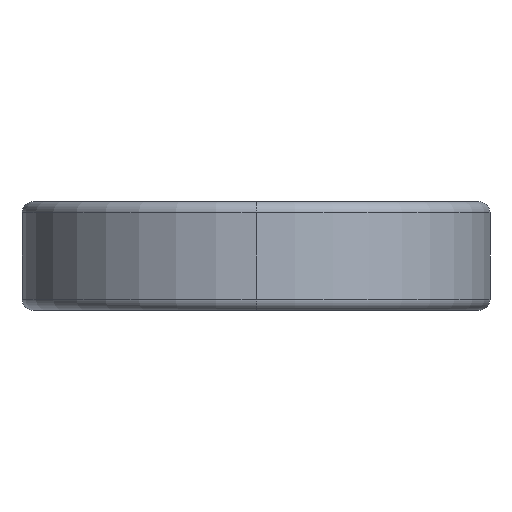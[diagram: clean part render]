
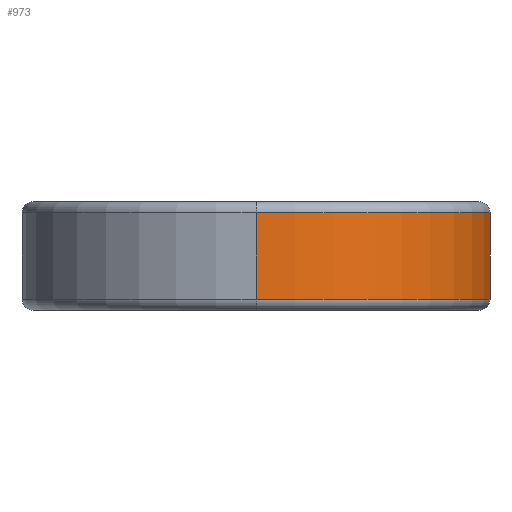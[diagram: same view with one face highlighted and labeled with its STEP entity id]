
A CAD part, left-side view. The second image highlights one B-rep face of the part: STEP entity #973.
In plain terms, the highlighted cylindrical face has radius 10.668 mm (diameter 21.336 mm), a partial arc.
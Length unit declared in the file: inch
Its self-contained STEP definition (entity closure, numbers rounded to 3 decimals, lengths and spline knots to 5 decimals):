
#16 = ORIENTED_EDGE ( 'NONE', *, *, #941, .F. ) ;
#33 = EDGE_CURVE ( 'NONE', #441, #615, #709, .T. ) ;
#49 = DIRECTION ( 'NONE',  ( -1., 0., 0. ) ) ;
#127 = CARTESIAN_POINT ( 'NONE',  ( -0.81309, -0.12194, 0.0775 ) ) ;
#135 = VECTOR ( 'NONE', #873, 39.37008 ) ;
#189 = DIRECTION ( 'NONE',  ( 0., 0., -1. ) ) ;
#251 = CARTESIAN_POINT ( 'NONE',  ( -0.81309, -0.12194, -0.0775 ) ) ;
#272 = AXIS2_PLACEMENT_3D ( 'NONE', #799, #640, #789 ) ;
#315 = EDGE_LOOP ( 'NONE', ( #711, #318, #765, #16 ) ) ;
#318 = ORIENTED_EDGE ( 'NONE', *, *, #33, .T. ) ;
#354 = CARTESIAN_POINT ( 'NONE',  ( -1.215, 0., 0.0775 ) ) ;
#373 = CIRCLE ( 'NONE', #403, 0.42 ) ;
#380 = CARTESIAN_POINT ( 'NONE',  ( -1.635, 0., 0.0775 ) ) ;
#396 = CYLINDRICAL_SURFACE ( 'NONE', #272, 0.42 ) ;
#403 = AXIS2_PLACEMENT_3D ( 'NONE', #665, #577, #49 ) ;
#405 = CIRCLE ( 'NONE', #1008, 0.42 ) ;
#441 = VERTEX_POINT ( 'NONE', #380 ) ;
#478 = VERTEX_POINT ( 'NONE', #127 ) ;
#493 = DIRECTION ( 'NONE',  ( 0., 0., -1. ) ) ;
#510 = VERTEX_POINT ( 'NONE', #251 ) ;
#564 = DIRECTION ( 'NONE',  ( -1., 0., 0. ) ) ;
#577 = DIRECTION ( 'NONE',  ( 0., 0., 1. ) ) ;
#615 = VERTEX_POINT ( 'NONE', #732 ) ;
#640 = DIRECTION ( 'NONE',  ( 0., 0., -1. ) ) ;
#665 = CARTESIAN_POINT ( 'NONE',  ( -1.215, 0., -0.0775 ) ) ;
#709 = LINE ( 'NONE', #855, #135 ) ;
#711 = ORIENTED_EDGE ( 'NONE', *, *, #841, .T. ) ;
#732 = CARTESIAN_POINT ( 'NONE',  ( -1.635, 0., -0.0775 ) ) ;
#734 = VECTOR ( 'NONE', #189, 39.37008 ) ;
#765 = ORIENTED_EDGE ( 'NONE', *, *, #998, .T. ) ;
#789 = DIRECTION ( 'NONE',  ( -1., 0., 0. ) ) ;
#799 = CARTESIAN_POINT ( 'NONE',  ( -1.215, 0., 0.0975 ) ) ;
#836 = FACE_OUTER_BOUND ( 'NONE', #315, .T. ) ;
#841 = EDGE_CURVE ( 'NONE', #478, #441, #405, .T. ) ;
#855 = CARTESIAN_POINT ( 'NONE',  ( -1.635, 0., 0.0975 ) ) ;
#873 = DIRECTION ( 'NONE',  ( 0., 0., -1. ) ) ;
#941 = EDGE_CURVE ( 'NONE', #478, #510, #983, .T. ) ;
#966 = CARTESIAN_POINT ( 'NONE',  ( -0.81309, -0.12194, 0.0975 ) ) ;
#973 = ADVANCED_FACE ( 'NONE', ( #836 ), #396, .T. ) ;
#983 = LINE ( 'NONE', #966, #734 ) ;
#998 = EDGE_CURVE ( 'NONE', #615, #510, #373, .T. ) ;
#1008 = AXIS2_PLACEMENT_3D ( 'NONE', #354, #493, #564 ) ;
